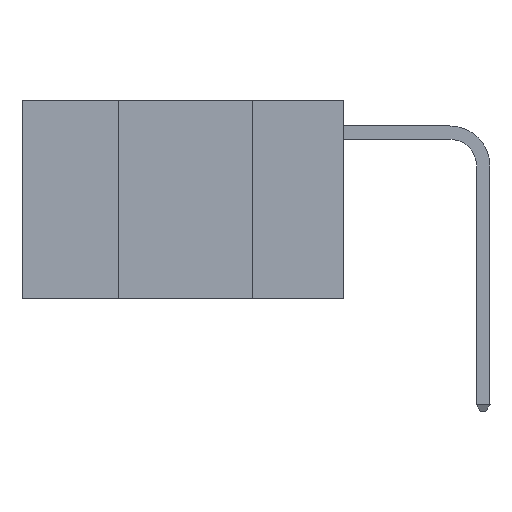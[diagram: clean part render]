
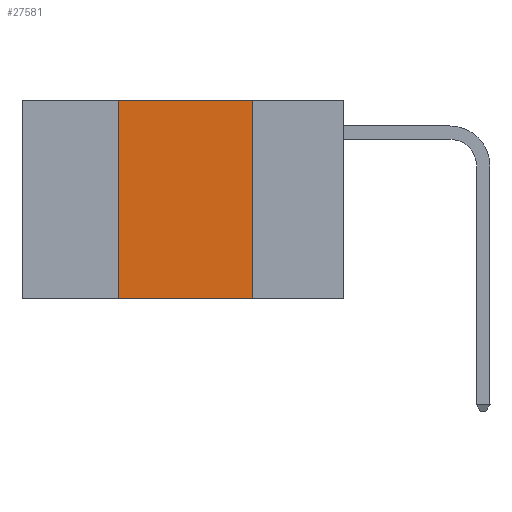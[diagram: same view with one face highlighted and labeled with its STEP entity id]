
A CAD part, left-side view. The second image highlights one B-rep face of the part: STEP entity #27581.
In plain terms, the highlighted planar face has unit normal (-1, 0, 0).
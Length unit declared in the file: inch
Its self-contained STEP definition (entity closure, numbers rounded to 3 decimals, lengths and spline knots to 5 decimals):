
#265 = ORIENTED_EDGE ( 'NONE', *, *, #1118, .T. ) ;
#543 = DIRECTION ( 'NONE',  ( 0., 0., 1. ) ) ;
#864 = ORIENTED_EDGE ( 'NONE', *, *, #4880, .F. ) ;
#1118 = EDGE_CURVE ( 'NONE', #25347, #8985, #5028, .T. ) ;
#1957 = ORIENTED_EDGE ( 'NONE', *, *, #10550, .F. ) ;
#2156 = VECTOR ( 'NONE', #5886, 39.37008 ) ;
#4421 = ORIENTED_EDGE ( 'NONE', *, *, #8094, .F. ) ;
#4426 = PLANE ( 'NONE',  #11710 ) ;
#4880 = EDGE_CURVE ( 'NONE', #7325, #21647, #17562, .T. ) ;
#5028 = LINE ( 'NONE', #16037, #23018 ) ;
#5886 = DIRECTION ( 'NONE',  ( 0., 0., -1. ) ) ;
#7325 = VERTEX_POINT ( 'NONE', #11406 ) ;
#8094 = EDGE_CURVE ( 'NONE', #25347, #7325, #10034, .T. ) ;
#8985 = VERTEX_POINT ( 'NONE', #14925 ) ;
#10034 = LINE ( 'NONE', #18639, #14645 ) ;
#10550 = EDGE_CURVE ( 'NONE', #21647, #8985, #14131, .T. ) ;
#11178 = CARTESIAN_POINT ( 'NONE',  ( 0., 0.6, 0. ) ) ;
#11406 = CARTESIAN_POINT ( 'NONE',  ( 0., 0.42, 0. ) ) ;
#11710 = AXIS2_PLACEMENT_3D ( 'NONE', #11178, #13459, #28195 ) ;
#13459 = DIRECTION ( 'NONE',  ( 1., 0., 0. ) ) ;
#14131 = LINE ( 'NONE', #23886, #2156 ) ;
#14645 = VECTOR ( 'NONE', #543, 39.37008 ) ;
#14925 = CARTESIAN_POINT ( 'NONE',  ( 0., 0.17, -0.37 ) ) ;
#15645 = DIRECTION ( 'NONE',  ( 0., -1., 0. ) ) ;
#16037 = CARTESIAN_POINT ( 'NONE',  ( 0., 0.6, -0.37 ) ) ;
#17562 = LINE ( 'NONE', #26325, #22833 ) ;
#18639 = CARTESIAN_POINT ( 'NONE',  ( 0., 0.42, 0. ) ) ;
#18797 = CARTESIAN_POINT ( 'NONE',  ( 0., 0.17, 0. ) ) ;
#20996 = FACE_OUTER_BOUND ( 'NONE', #28344, .T. ) ;
#21647 = VERTEX_POINT ( 'NONE', #18797 ) ;
#22833 = VECTOR ( 'NONE', #28576, 39.37008 ) ;
#23018 = VECTOR ( 'NONE', #15645, 39.37008 ) ;
#23886 = CARTESIAN_POINT ( 'NONE',  ( 0., 0.17, 0. ) ) ;
#25347 = VERTEX_POINT ( 'NONE', #27615 ) ;
#26325 = CARTESIAN_POINT ( 'NONE',  ( 0., 0.6, 0. ) ) ;
#27581 = ADVANCED_FACE ( 'NONE', ( #20996 ), #4426, .F. ) ;
#27615 = CARTESIAN_POINT ( 'NONE',  ( 0., 0.42, -0.37 ) ) ;
#28195 = DIRECTION ( 'NONE',  ( 0., 0., -1. ) ) ;
#28344 = EDGE_LOOP ( 'NONE', ( #1957, #864, #4421, #265 ) ) ;
#28576 = DIRECTION ( 'NONE',  ( 0., -1., 0. ) ) ;
